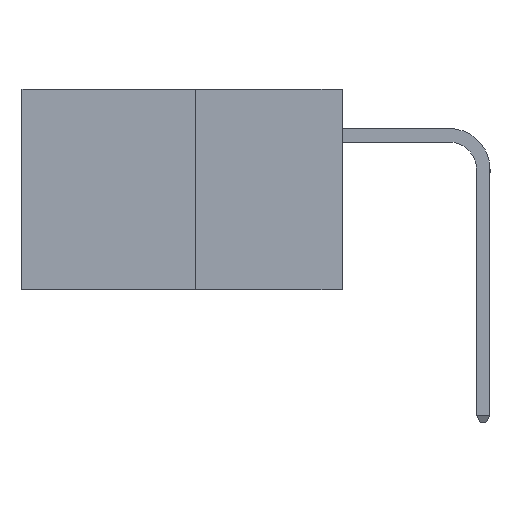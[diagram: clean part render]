
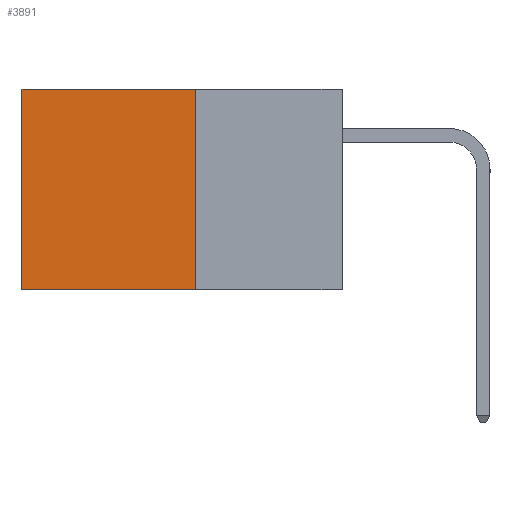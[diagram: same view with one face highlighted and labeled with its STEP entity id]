
A CAD part, left-side view. The second image highlights one B-rep face of the part: STEP entity #3891.
In plain terms, the highlighted planar face has unit normal (-1, 0, 0).
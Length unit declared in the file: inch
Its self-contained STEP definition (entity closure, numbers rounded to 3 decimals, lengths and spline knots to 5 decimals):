
#248 = DIRECTION ( 'NONE',  ( 0., 0., -1. ) ) ;
#545 = EDGE_CURVE ( 'NONE', #10095, #2912, #6942, .T. ) ;
#704 = DIRECTION ( 'NONE',  ( 0., 1., 0. ) ) ;
#1253 = DIRECTION ( 'NONE',  ( 1., 0., 0. ) ) ;
#1850 = ORIENTED_EDGE ( 'NONE', *, *, #4087, .T. ) ;
#1862 = LINE ( 'NONE', #10724, #10820 ) ;
#2163 = ORIENTED_EDGE ( 'NONE', *, *, #10391, .T. ) ;
#2881 = DIRECTION ( 'NONE',  ( 0., 0., -1. ) ) ;
#2912 = VERTEX_POINT ( 'NONE', #7907 ) ;
#3618 = CARTESIAN_POINT ( 'NONE',  ( 0.277, 0.27, -0.37 ) ) ;
#3891 = ADVANCED_FACE ( 'NONE', ( #10684 ), #10838, .F. ) ;
#4006 = VECTOR ( 'NONE', #2881, 39.37008 ) ;
#4087 = EDGE_CURVE ( 'NONE', #9229, #2912, #1862, .T. ) ;
#4789 = EDGE_LOOP ( 'NONE', ( #1850, #8832, #11063, #2163 ) ) ;
#4851 = VECTOR ( 'NONE', #5477, 39.37008 ) ;
#5477 = DIRECTION ( 'NONE',  ( 0., 1., 0. ) ) ;
#5717 = AXIS2_PLACEMENT_3D ( 'NONE', #3618, #1253, #248 ) ;
#6056 = LINE ( 'NONE', #7264, #4006 ) ;
#6302 = CARTESIAN_POINT ( 'NONE',  ( 0.277, 0.27, 0. ) ) ;
#6676 = VECTOR ( 'NONE', #704, 39.37008 ) ;
#6817 = CARTESIAN_POINT ( 'NONE',  ( 0.277, 0.27, -0.37 ) ) ;
#6942 = LINE ( 'NONE', #6817, #6676 ) ;
#7264 = CARTESIAN_POINT ( 'NONE',  ( 0.277, 0.27, -0.37 ) ) ;
#7907 = CARTESIAN_POINT ( 'NONE',  ( 0.277, 0.59, -0.37 ) ) ;
#8317 = CARTESIAN_POINT ( 'NONE',  ( 0.277, 0.27, 0. ) ) ;
#8832 = ORIENTED_EDGE ( 'NONE', *, *, #545, .F. ) ;
#8903 = CARTESIAN_POINT ( 'NONE',  ( 0.277, 0.59, 0. ) ) ;
#9229 = VERTEX_POINT ( 'NONE', #8903 ) ;
#9331 = LINE ( 'NONE', #6302, #4851 ) ;
#9464 = VERTEX_POINT ( 'NONE', #8317 ) ;
#10095 = VERTEX_POINT ( 'NONE', #11024 ) ;
#10391 = EDGE_CURVE ( 'NONE', #9464, #9229, #9331, .T. ) ;
#10538 = EDGE_CURVE ( 'NONE', #9464, #10095, #6056, .T. ) ;
#10684 = FACE_OUTER_BOUND ( 'NONE', #4789, .T. ) ;
#10724 = CARTESIAN_POINT ( 'NONE',  ( 0.277, 0.59, -0.37 ) ) ;
#10820 = VECTOR ( 'NONE', #10834, 39.37008 ) ;
#10834 = DIRECTION ( 'NONE',  ( 0., 0., -1. ) ) ;
#10838 = PLANE ( 'NONE',  #5717 ) ;
#11024 = CARTESIAN_POINT ( 'NONE',  ( 0.277, 0.27, -0.37 ) ) ;
#11063 = ORIENTED_EDGE ( 'NONE', *, *, #10538, .F. ) ;
